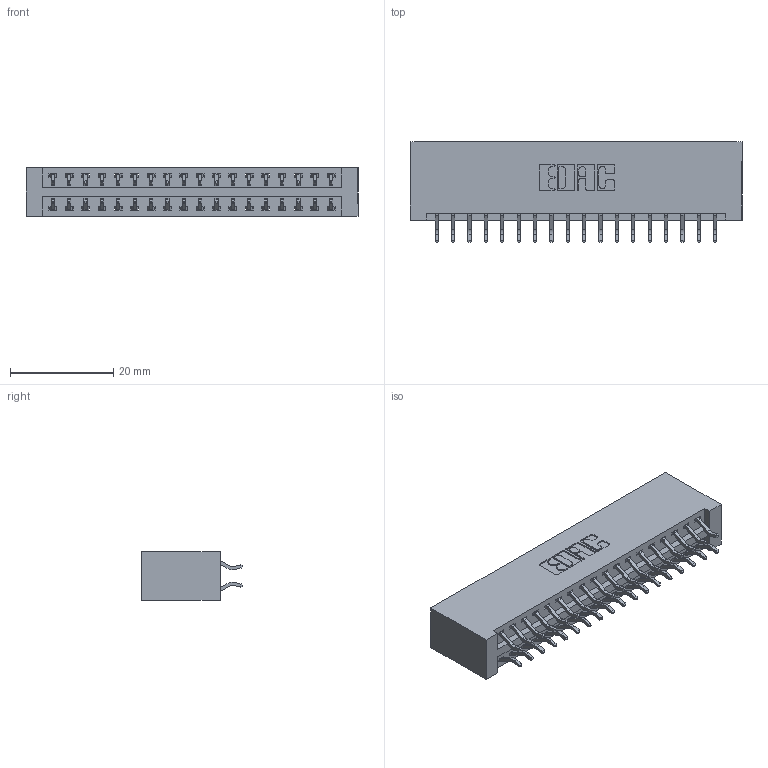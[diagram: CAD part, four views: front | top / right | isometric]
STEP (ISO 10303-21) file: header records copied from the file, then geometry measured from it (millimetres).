
FILE_DESCRIPTION (( 'STEP AP203' ), '1' );
FILE_NAME ('346-036-556-201.STEP', '2022-05-19T22:04:28', ( '' ), ( '' ), 'SwSTEP 2.0', 'SolidWorks 2020', '' );
FILE_SCHEMA (( 'CONFIG_CONTROL_DESIGN' ));
Length unit declared in the file: inch
Products named in the file (3): 345-292-001_556 Tail; 346-036-556-201; 346 Part_No Mounting Lugs
Assembly tree (37 placements, depth 2):
  346-036-556-201
    346 Part_No Mounting Lugs
    345-292-001_556 Tail  x36
Bounding box: 64.39 x 19.57 x 9.4 mm (x, y, z)
Volume: 6664.2 mm3; surface area: 8912.9 mm2
Topology: 37 solids, 37 shells, 2202 faces, 6533 edges, 4306 vertices
Faces by surface type: plane 1476, cylinder 726
Entity records: 14921 total; most frequent: CARTESIAN_POINT 2504, ORIENTED_EDGE 2426, DIRECTION 2241, EDGE_CURVE 1213, VECTOR 1009, LINE 1009, VERTEX_POINT 806, AXIS2_PLACEMENT_3D 616
